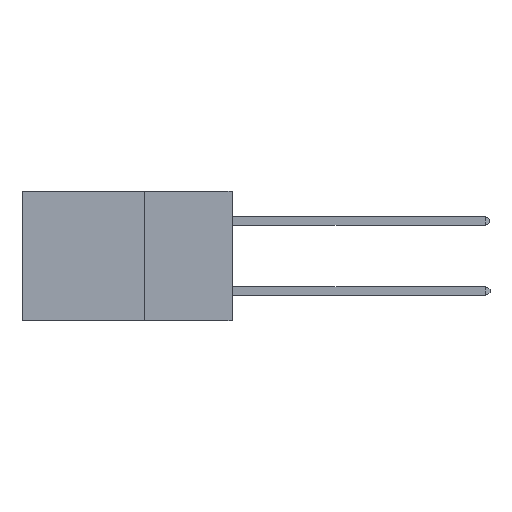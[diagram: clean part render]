
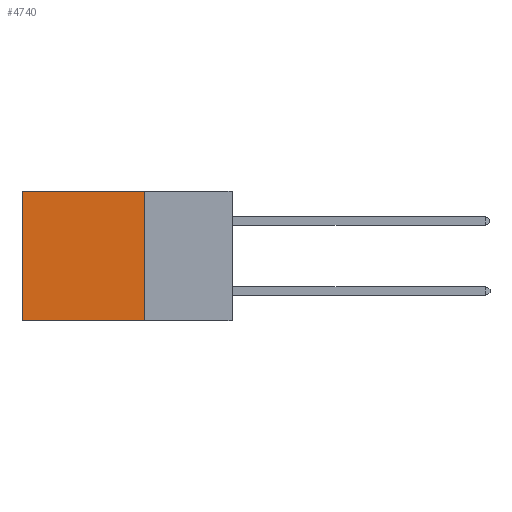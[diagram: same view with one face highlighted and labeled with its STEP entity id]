
A CAD part, left-side view. The second image highlights one B-rep face of the part: STEP entity #4740.
In plain terms, the highlighted planar face has unit normal (-1, 0, 0).
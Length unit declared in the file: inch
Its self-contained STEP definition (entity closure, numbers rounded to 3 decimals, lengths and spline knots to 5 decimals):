
#1218 = VECTOR ( 'NONE', #10203, 39.37008 ) ;
#2278 = LINE ( 'NONE', #5988, #10229 ) ;
#3282 = VERTEX_POINT ( 'NONE', #7752 ) ;
#4723 = CARTESIAN_POINT ( 'NONE',  ( 0.2875, 0.6, -0.37 ) ) ;
#4740 = ADVANCED_FACE ( 'NONE', ( #8673 ), #5740, .F. ) ;
#5740 = PLANE ( 'NONE',  #19770 ) ;
#5988 = CARTESIAN_POINT ( 'NONE',  ( 0.2875, 0.25, 0. ) ) ;
#6851 = LINE ( 'NONE', #9624, #11808 ) ;
#7236 = ORIENTED_EDGE ( 'NONE', *, *, #8757, .T. ) ;
#7752 = CARTESIAN_POINT ( 'NONE',  ( 0.2875, 0.25, 0. ) ) ;
#7909 = CARTESIAN_POINT ( 'NONE',  ( 0.2875, 0.25, 0. ) ) ;
#8666 = VECTOR ( 'NONE', #17815, 39.37008 ) ;
#8673 = FACE_OUTER_BOUND ( 'NONE', #20545, .T. ) ;
#8757 = EDGE_CURVE ( 'NONE', #11644, #20525, #18467, .T. ) ;
#9136 = DIRECTION ( 'NONE',  ( 0., 0., -1. ) ) ;
#9624 = CARTESIAN_POINT ( 'NONE',  ( 0.2875, 0.25, -0.37 ) ) ;
#9797 = ORIENTED_EDGE ( 'NONE', *, *, #15654, .F. ) ;
#10203 = DIRECTION ( 'NONE',  ( 0., 0., -1. ) ) ;
#10229 = VECTOR ( 'NONE', #19262, 39.37008 ) ;
#11381 = CARTESIAN_POINT ( 'NONE',  ( 0.2875, 0.6, 0. ) ) ;
#11644 = VERTEX_POINT ( 'NONE', #11381 ) ;
#11808 = VECTOR ( 'NONE', #17923, 39.37008 ) ;
#11899 = VERTEX_POINT ( 'NONE', #20310 ) ;
#14882 = ORIENTED_EDGE ( 'NONE', *, *, #16708, .T. ) ;
#15654 = EDGE_CURVE ( 'NONE', #11899, #20525, #6851, .T. ) ;
#16606 = EDGE_CURVE ( 'NONE', #3282, #11899, #2278, .T. ) ;
#16708 = EDGE_CURVE ( 'NONE', #3282, #11644, #21308, .T. ) ;
#17240 = ORIENTED_EDGE ( 'NONE', *, *, #16606, .F. ) ;
#17291 = CARTESIAN_POINT ( 'NONE',  ( 0.2875, 0.25, 0. ) ) ;
#17815 = DIRECTION ( 'NONE',  ( 0., 1., 0. ) ) ;
#17923 = DIRECTION ( 'NONE',  ( 0., 1., 0. ) ) ;
#18467 = LINE ( 'NONE', #20068, #1218 ) ;
#19011 = DIRECTION ( 'NONE',  ( 1., 0., 0. ) ) ;
#19262 = DIRECTION ( 'NONE',  ( 0., 0., -1. ) ) ;
#19770 = AXIS2_PLACEMENT_3D ( 'NONE', #17291, #19011, #9136 ) ;
#20068 = CARTESIAN_POINT ( 'NONE',  ( 0.2875, 0.6, 0. ) ) ;
#20310 = CARTESIAN_POINT ( 'NONE',  ( 0.2875, 0.25, -0.37 ) ) ;
#20525 = VERTEX_POINT ( 'NONE', #4723 ) ;
#20545 = EDGE_LOOP ( 'NONE', ( #7236, #9797, #17240, #14882 ) ) ;
#21308 = LINE ( 'NONE', #7909, #8666 ) ;
